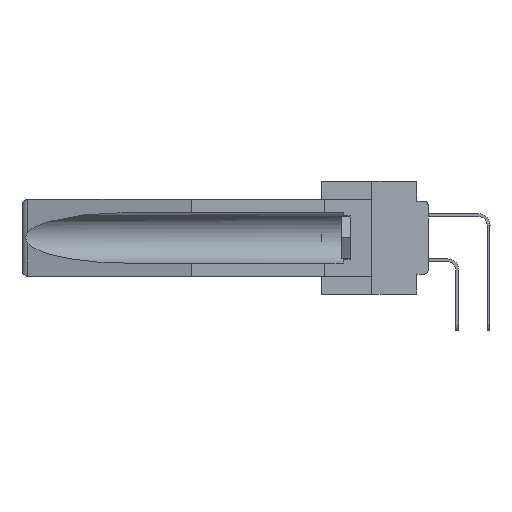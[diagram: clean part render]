
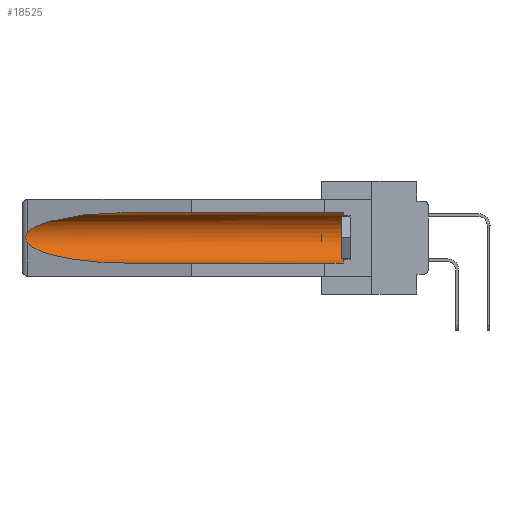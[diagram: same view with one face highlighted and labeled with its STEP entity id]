
A CAD part, left-side view. The second image highlights one B-rep face of the part: STEP entity #18525.
In plain terms, the highlighted cylindrical face has radius 2.857 mm (diameter 5.715 mm), a partial arc.
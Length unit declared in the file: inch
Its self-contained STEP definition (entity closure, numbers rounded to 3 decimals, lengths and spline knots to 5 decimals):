
#1548 = ORIENTED_EDGE ( 'NONE', *, *, #12283, .T. ) ;
#1959 = EDGE_CURVE ( 'NONE', #10753, #34043, #35904, .T. ) ;
#2320 = ORIENTED_EDGE ( 'NONE', *, *, #29327, .T. ) ;
#2323 = CARTESIAN_POINT ( 'NONE',  ( 0.25451, 1.48313, -0.09465 ) ) ;
#3759 = AXIS2_PLACEMENT_3D ( 'NONE', #4378, #37594, #17790 ) ;
#4378 = CARTESIAN_POINT ( 'NONE',  ( 0.155, -0.30754, -0.1715 ) ) ;
#4494 = EDGE_CURVE ( 'NONE', #12611, #10753, #23667, .T. ) ;
#6098 = CARTESIAN_POINT ( 'NONE',  ( 0.26597, 1.52961, -0.15275 ) ) ;
#9057 = VERTEX_POINT ( 'NONE', #25898 ) ;
#9304 = AXIS2_PLACEMENT_3D ( 'NONE', #14578, #11540, #11248 ) ;
#10753 = VERTEX_POINT ( 'NONE', #21628 ) ;
#11248 = DIRECTION ( 'NONE',  ( 0., 0., 1. ) ) ;
#11540 = DIRECTION ( 'NONE',  ( 0., -1., 0. ) ) ;
#12283 = EDGE_CURVE ( 'NONE', #29029, #26224, #32985, .T. ) ;
#12611 = VERTEX_POINT ( 'NONE', #14241 ) ;
#13711 = ORIENTED_EDGE ( 'NONE', *, *, #22308, .T. ) ;
#13749 = ORIENTED_EDGE ( 'NONE', *, *, #1959, .T. ) ;
#13817 = CARTESIAN_POINT ( 'NONE',  ( 0.155, 1.07973, -0.284 ) ) ;
#14241 = CARTESIAN_POINT ( 'NONE',  ( 0.26537, 1.52718, -0.14972 ) ) ;
#14578 = CARTESIAN_POINT ( 'NONE',  ( 0.155, 0.126, -0.1715 ) ) ;
#15790 = CIRCLE ( 'NONE', #9304, 0.1125 ) ;
#15929 = CARTESIAN_POINT ( 'NONE',  ( 0.26537, 1.52718, -0.19328 ) ) ;
#16910 = CARTESIAN_POINT ( 'NONE',  ( 0.155, 1.07973, -0.284 ) ) ;
#17790 = DIRECTION ( 'NONE',  ( 0., 0., 1. ) ) ;
#18122 = CYLINDRICAL_SURFACE ( 'NONE', #3759, 0.1125 ) ;
#18525 = ADVANCED_FACE ( 'NONE', ( #27931 ), #18122, .F. ) ;
#18604 = CARTESIAN_POINT ( 'NONE',  ( 0.26537, 1.52718, -0.14972 ) ) ;
#19096 = CARTESIAN_POINT ( 'NONE',  ( 0.26597, 1.5296, -0.19026 ) ) ;
#19538 = CARTESIAN_POINT ( 'NONE',  ( 0.2673, 1.53269, -0.17917 ) ) ;
#20520 =( BOUNDED_CURVE ( )  B_SPLINE_CURVE ( 3, ( #41729, #42321, #2323, #18604 ),
 .UNSPECIFIED., .F., .F. ) 
 B_SPLINE_CURVE_WITH_KNOTS ( ( 4, 4 ),
 ( 4.71239, 6.08839 ),
 .UNSPECIFIED. ) 
 CURVE ( )  GEOMETRIC_REPRESENTATION_ITEM ( )  RATIONAL_B_SPLINE_CURVE ( ( 1., 0.848, 0.848, 1. ) ) 
 REPRESENTATION_ITEM ( '' )  );
#21628 = CARTESIAN_POINT ( 'NONE',  ( 0.26537, 1.52718, -0.19328 ) ) ;
#22308 = EDGE_CURVE ( 'NONE', #26224, #12611, #20520, .T. ) ;
#22547 = CARTESIAN_POINT ( 'NONE',  ( 0.26537, 1.52718, -0.14972 ) ) ;
#23667 = B_SPLINE_CURVE_WITH_KNOTS ( 'NONE', 3,
 ( #22547, #6098, #35578, #35715, #38878, #28905, #19538, #30500, #19096, #15929 ),
 .UNSPECIFIED., .F., .F.,
 ( 4, 2, 2, 2, 4 ),
 ( 0., 0.00029, 0.00058, 0.00087, 0.00117 ),
 .UNSPECIFIED. ) ;
#24131 = EDGE_CURVE ( 'NONE', #9057, #34043, #41243, .T. ) ;
#25898 = CARTESIAN_POINT ( 'NONE',  ( 0.155, 0.126, -0.284 ) ) ;
#26224 = VERTEX_POINT ( 'NONE', #31274 ) ;
#27338 = CARTESIAN_POINT ( 'NONE',  ( 0.26537, 1.52718, -0.19328 ) ) ;
#27931 = FACE_OUTER_BOUND ( 'NONE', #31464, .T. ) ;
#28563 = DIRECTION ( 'NONE',  ( 0., 1., 0. ) ) ;
#28905 = CARTESIAN_POINT ( 'NONE',  ( 0.2675, 1.53308, -0.17534 ) ) ;
#29029 = VERTEX_POINT ( 'NONE', #29607 ) ;
#29327 = EDGE_CURVE ( 'NONE', #9057, #29029, #15790, .T. ) ;
#29374 = VECTOR ( 'NONE', #35186, 39.37008 ) ;
#29554 = ORIENTED_EDGE ( 'NONE', *, *, #24131, .F. ) ;
#29607 = CARTESIAN_POINT ( 'NONE',  ( 0.155, 0.126, -0.059 ) ) ;
#30500 = CARTESIAN_POINT ( 'NONE',  ( 0.26655, 1.53094, -0.18657 ) ) ;
#31274 = CARTESIAN_POINT ( 'NONE',  ( 0.155, 1.07973, -0.059 ) ) ;
#31464 = EDGE_LOOP ( 'NONE', ( #13711, #39410, #13749, #29554, #2320, #1548 ) ) ;
#31939 = VECTOR ( 'NONE', #28563, 39.37008 ) ;
#32144 = CARTESIAN_POINT ( 'NONE',  ( 0.155, -0.30754, -0.059 ) ) ;
#32985 = LINE ( 'NONE', #32144, #29374 ) ;
#33563 = CARTESIAN_POINT ( 'NONE',  ( 0.25451, 1.48313, -0.24835 ) ) ;
#33989 = CARTESIAN_POINT ( 'NONE',  ( 0.21114, 1.30732, -0.284 ) ) ;
#34043 = VERTEX_POINT ( 'NONE', #16910 ) ;
#35186 = DIRECTION ( 'NONE',  ( 0., 1., 0. ) ) ;
#35578 = CARTESIAN_POINT ( 'NONE',  ( 0.26654, 1.53092, -0.15636 ) ) ;
#35715 = CARTESIAN_POINT ( 'NONE',  ( 0.2673, 1.5327, -0.16383 ) ) ;
#35904 =( BOUNDED_CURVE ( )  B_SPLINE_CURVE ( 3, ( #27338, #33563, #33989, #13817 ),
 .UNSPECIFIED., .F., .F. ) 
 B_SPLINE_CURVE_WITH_KNOTS ( ( 4, 4 ),
 ( 0.1948, 1.5708 ),
 .UNSPECIFIED. ) 
 CURVE ( )  GEOMETRIC_REPRESENTATION_ITEM ( )  RATIONAL_B_SPLINE_CURVE ( ( 1., 0.848, 0.848, 1. ) ) 
 REPRESENTATION_ITEM ( '' )  );
#37594 = DIRECTION ( 'NONE',  ( 0., 1., 0. ) ) ;
#38878 = CARTESIAN_POINT ( 'NONE',  ( 0.2675, 1.53308, -0.16763 ) ) ;
#39410 = ORIENTED_EDGE ( 'NONE', *, *, #4494, .T. ) ;
#41243 = LINE ( 'NONE', #42176, #31939 ) ;
#41729 = CARTESIAN_POINT ( 'NONE',  ( 0.155, 1.07973, -0.059 ) ) ;
#42176 = CARTESIAN_POINT ( 'NONE',  ( 0.155, -0.30754, -0.284 ) ) ;
#42321 = CARTESIAN_POINT ( 'NONE',  ( 0.21114, 1.30732, -0.059 ) ) ;
